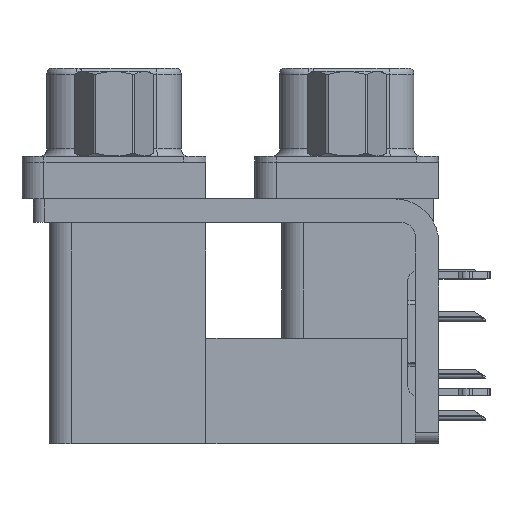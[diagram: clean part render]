
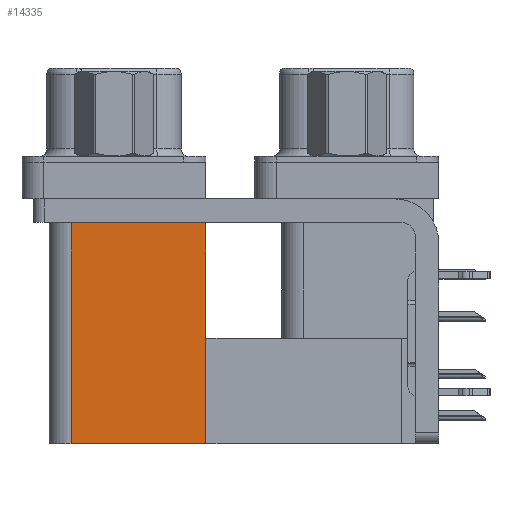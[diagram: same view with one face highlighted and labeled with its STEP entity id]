
A CAD part, left-side view. The second image highlights one B-rep face of the part: STEP entity #14335.
In plain terms, the highlighted planar face has unit normal (-1, 0, 0).
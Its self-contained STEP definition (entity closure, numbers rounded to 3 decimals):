
#79 = CARTESIAN_POINT ( 'NONE',  ( 3.7, 9.6, -19.2 ) ) ;
#2982 = EDGE_CURVE ( 'NONE', #37567, #38639, #25494, .T. ) ;
#3610 = ORIENTED_EDGE ( 'NONE', *, *, #2982, .T. ) ;
#3776 = ORIENTED_EDGE ( 'NONE', *, *, #26189, .F. ) ;
#4882 = LINE ( 'NONE', #8027, #34156 ) ;
#6584 = EDGE_LOOP ( 'NONE', ( #27551, #46540, #3776, #3610 ) ) ;
#6868 = FACE_OUTER_BOUND ( 'NONE', #6584, .T. ) ;
#6917 = VECTOR ( 'NONE', #18487, 1000. ) ;
#7342 = PLANE ( 'NONE',  #29611 ) ;
#8027 = CARTESIAN_POINT ( 'NONE',  ( 3.7, 9.6, -19.2 ) ) ;
#8200 = EDGE_CURVE ( 'NONE', #38639, #27507, #18250, .T. ) ;
#11884 = DIRECTION ( 'NONE',  ( 0., 1., 0. ) ) ;
#14335 = ADVANCED_FACE ( 'NONE', ( #6868 ), #7342, .F. ) ;
#16166 = LINE ( 'NONE', #27748, #27907 ) ;
#18250 = LINE ( 'NONE', #47259, #6917 ) ;
#18487 = DIRECTION ( 'NONE',  ( 0., 1., 0. ) ) ;
#24117 = DIRECTION ( 'NONE',  ( 0., 0., 1. ) ) ;
#25431 = EDGE_CURVE ( 'NONE', #44428, #27507, #16166, .T. ) ;
#25494 = LINE ( 'NONE', #35688, #43901 ) ;
#26171 = DIRECTION ( 'NONE',  ( 1., 0., 0. ) ) ;
#26189 = EDGE_CURVE ( 'NONE', #37567, #44428, #4882, .T. ) ;
#27507 = VERTEX_POINT ( 'NONE', #32068 ) ;
#27551 = ORIENTED_EDGE ( 'NONE', *, *, #8200, .T. ) ;
#27748 = CARTESIAN_POINT ( 'NONE',  ( 3.7, 18.8, -19.2 ) ) ;
#27907 = VECTOR ( 'NONE', #24117, 1000. ) ;
#28373 = CARTESIAN_POINT ( 'NONE',  ( 3.7, 9.6, -19.2 ) ) ;
#29611 = AXIS2_PLACEMENT_3D ( 'NONE', #79, #26171, #43829 ) ;
#32068 = CARTESIAN_POINT ( 'NONE',  ( 3.7, 18.8, -2.5 ) ) ;
#32534 = DIRECTION ( 'NONE',  ( 0., 0., 1. ) ) ;
#34156 = VECTOR ( 'NONE', #11884, 1000. ) ;
#35688 = CARTESIAN_POINT ( 'NONE',  ( 3.7, 9.6, -19.2 ) ) ;
#37567 = VERTEX_POINT ( 'NONE', #28373 ) ;
#37601 = CARTESIAN_POINT ( 'NONE',  ( 3.7, 9.6, -2.5 ) ) ;
#38053 = CARTESIAN_POINT ( 'NONE',  ( 3.7, 18.8, -19.2 ) ) ;
#38639 = VERTEX_POINT ( 'NONE', #37601 ) ;
#43829 = DIRECTION ( 'NONE',  ( 0., 0., -1. ) ) ;
#43901 = VECTOR ( 'NONE', #32534, 1000. ) ;
#44428 = VERTEX_POINT ( 'NONE', #38053 ) ;
#46540 = ORIENTED_EDGE ( 'NONE', *, *, #25431, .F. ) ;
#47259 = CARTESIAN_POINT ( 'NONE',  ( 3.7, 9.6, -2.5 ) ) ;
